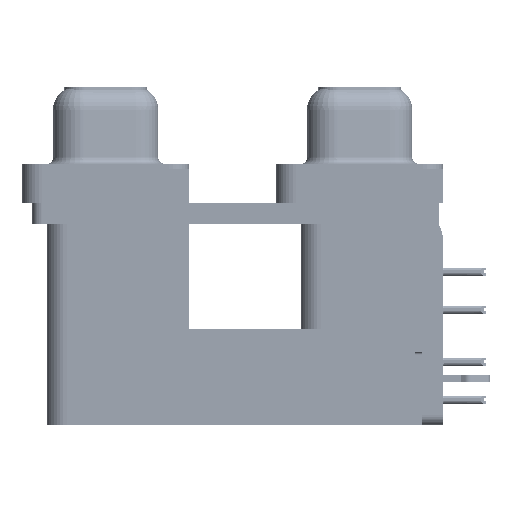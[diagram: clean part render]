
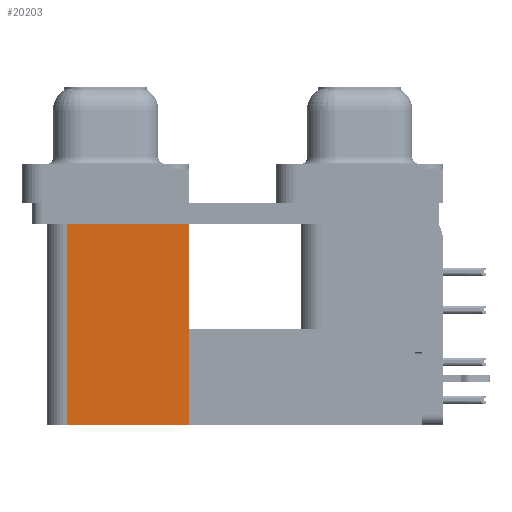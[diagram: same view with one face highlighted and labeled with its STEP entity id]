
A CAD part, left-side view. The second image highlights one B-rep face of the part: STEP entity #20203.
In plain terms, the highlighted planar face has unit normal (-1, 0, 0).
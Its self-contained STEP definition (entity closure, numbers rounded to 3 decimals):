
#1880 = DIRECTION ( 'NONE',  ( 0., 1., 0. ) ) ;
#2345 = EDGE_CURVE ( 'NONE', #46672, #12593, #22437, .T. ) ;
#8150 = CARTESIAN_POINT ( 'NONE',  ( 3.7, 21.975, -2.5 ) ) ;
#9655 = ORIENTED_EDGE ( 'NONE', *, *, #13950, .T. ) ;
#11019 = CARTESIAN_POINT ( 'NONE',  ( 3.7, 12.775, -2.5 ) ) ;
#11799 = LINE ( 'NONE', #35411, #48518 ) ;
#12593 = VERTEX_POINT ( 'NONE', #8150 ) ;
#13712 = CARTESIAN_POINT ( 'NONE',  ( 3.7, 21.975, -19.2 ) ) ;
#13950 = EDGE_CURVE ( 'NONE', #40418, #12593, #20409, .T. ) ;
#18916 = CARTESIAN_POINT ( 'NONE',  ( 3.7, 12.775, -19.2 ) ) ;
#20203 = ADVANCED_FACE ( 'NONE', ( #21867 ), #53976, .F. ) ;
#20409 = LINE ( 'NONE', #11019, #20501 ) ;
#20501 = VECTOR ( 'NONE', #1880, 1000. ) ;
#21255 = DIRECTION ( 'NONE',  ( 0., 1., 0. ) ) ;
#21867 = FACE_OUTER_BOUND ( 'NONE', #52111, .T. ) ;
#22437 = LINE ( 'NONE', #41203, #34240 ) ;
#23177 = ORIENTED_EDGE ( 'NONE', *, *, #2345, .F. ) ;
#25545 = ORIENTED_EDGE ( 'NONE', *, *, #37428, .F. ) ;
#26702 = CARTESIAN_POINT ( 'NONE',  ( 3.7, 12.775, -19.2 ) ) ;
#29784 = DIRECTION ( 'NONE',  ( 0., 0., 1. ) ) ;
#30269 = DIRECTION ( 'NONE',  ( 0., 1., 0. ) ) ;
#33999 = AXIS2_PLACEMENT_3D ( 'NONE', #26702, #40325, #21255 ) ;
#34240 = VECTOR ( 'NONE', #36652, 1000. ) ;
#35411 = CARTESIAN_POINT ( 'NONE',  ( 3.7, 12.775, -19.2 ) ) ;
#36652 = DIRECTION ( 'NONE',  ( 0., 0., 1. ) ) ;
#37428 = EDGE_CURVE ( 'NONE', #43805, #46672, #11799, .T. ) ;
#40325 = DIRECTION ( 'NONE',  ( 1., 0., 0. ) ) ;
#40418 = VERTEX_POINT ( 'NONE', #49522 ) ;
#41203 = CARTESIAN_POINT ( 'NONE',  ( 3.7, 21.975, -19.2 ) ) ;
#43805 = VERTEX_POINT ( 'NONE', #18916 ) ;
#46672 = VERTEX_POINT ( 'NONE', #13712 ) ;
#48518 = VECTOR ( 'NONE', #30269, 1000. ) ;
#49402 = ORIENTED_EDGE ( 'NONE', *, *, #55217, .T. ) ;
#49522 = CARTESIAN_POINT ( 'NONE',  ( 3.7, 12.775, -2.5 ) ) ;
#52111 = EDGE_LOOP ( 'NONE', ( #9655, #23177, #25545, #49402 ) ) ;
#52823 = LINE ( 'NONE', #58261, #58788 ) ;
#53976 = PLANE ( 'NONE',  #33999 ) ;
#55217 = EDGE_CURVE ( 'NONE', #43805, #40418, #52823, .T. ) ;
#58261 = CARTESIAN_POINT ( 'NONE',  ( 3.7, 12.775, -19.2 ) ) ;
#58788 = VECTOR ( 'NONE', #29784, 1000. ) ;
